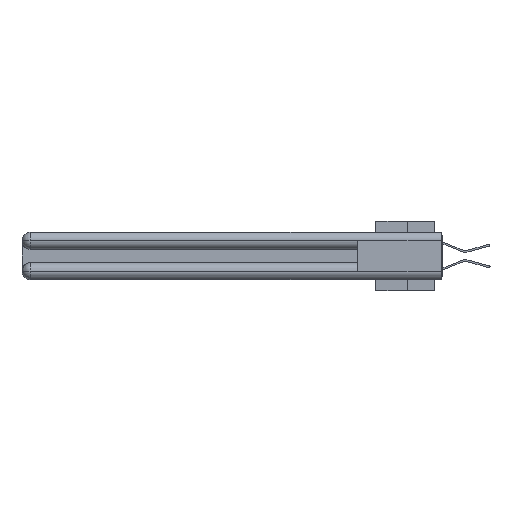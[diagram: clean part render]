
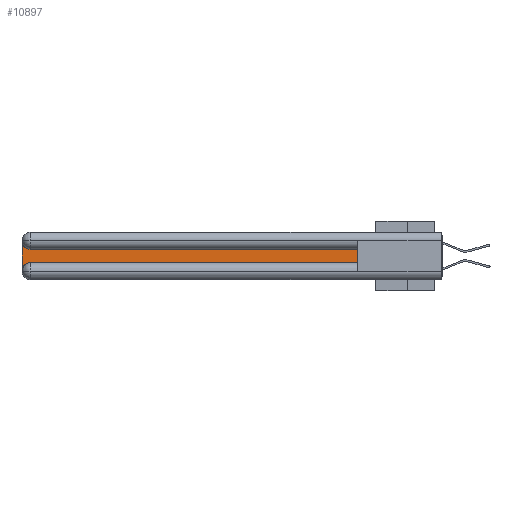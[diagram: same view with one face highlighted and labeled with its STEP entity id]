
A CAD part, left-side view. The second image highlights one B-rep face of the part: STEP entity #10897.
In plain terms, the highlighted planar face has unit normal (-1, 0, 0).
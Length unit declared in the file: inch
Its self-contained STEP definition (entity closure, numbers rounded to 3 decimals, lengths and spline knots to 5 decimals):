
#558 = PLANE ( 'NONE',  #18155 ) ;
#804 = DIRECTION ( 'NONE',  ( 1., 0., 0. ) ) ;
#1909 = VECTOR ( 'NONE', #27514, 39.37008 ) ;
#1958 = DIRECTION ( 'NONE',  ( 1., 0., 0. ) ) ;
#2050 = AXIS2_PLACEMENT_3D ( 'NONE', #28147, #11711, #31362 ) ;
#2185 = CARTESIAN_POINT ( 'NONE',  ( 0.075, 2.94, -0.0625 ) ) ;
#2773 = LINE ( 'NONE', #30263, #1909 ) ;
#3447 = DIRECTION ( 'NONE',  ( 0., 0., -1. ) ) ;
#4898 = CARTESIAN_POINT ( 'NONE',  ( 0.075, 2.94, -0.2175 ) ) ;
#7328 = DIRECTION ( 'NONE',  ( 0., -1., 0. ) ) ;
#7386 = CARTESIAN_POINT ( 'NONE',  ( 0.075, 0.6, -0.1225 ) ) ;
#7410 = CARTESIAN_POINT ( 'NONE',  ( 0.075, 2.94, -0.1225 ) ) ;
#7821 = CARTESIAN_POINT ( 'NONE',  ( 0.075, 0.6, -0.2175 ) ) ;
#8546 = EDGE_CURVE ( 'NONE', #30610, #24646, #12471, .T. ) ;
#9130 = VECTOR ( 'NONE', #7328, 39.37008 ) ;
#10398 = LINE ( 'NONE', #18314, #9130 ) ;
#10419 = ORIENTED_EDGE ( 'NONE', *, *, #33603, .T. ) ;
#10897 = ADVANCED_FACE ( 'NONE', ( #31747 ), #558, .F. ) ;
#11254 = EDGE_CURVE ( 'NONE', #23061, #30610, #17925, .T. ) ;
#11711 = DIRECTION ( 'NONE',  ( 1., 0., 0. ) ) ;
#12378 = ORIENTED_EDGE ( 'NONE', *, *, #11254, .T. ) ;
#12471 = CIRCLE ( 'NONE', #2050, 0.06 ) ;
#13074 = CARTESIAN_POINT ( 'NONE',  ( 0.075, 3., -0.2175 ) ) ;
#13587 = ORIENTED_EDGE ( 'NONE', *, *, #8546, .T. ) ;
#14089 = VECTOR ( 'NONE', #21341, 39.37008 ) ;
#15757 = AXIS2_PLACEMENT_3D ( 'NONE', #2185, #1958, #32156 ) ;
#16210 = DIRECTION ( 'NONE',  ( 0., 0., 1. ) ) ;
#16212 = VERTEX_POINT ( 'NONE', #7410 ) ;
#16827 = EDGE_CURVE ( 'NONE', #16212, #23061, #25061, .T. ) ;
#17368 = EDGE_CURVE ( 'NONE', #24646, #25975, #10398, .T. ) ;
#17925 = LINE ( 'NONE', #13074, #14089 ) ;
#18155 = AXIS2_PLACEMENT_3D ( 'NONE', #28028, #804, #3447 ) ;
#18314 = CARTESIAN_POINT ( 'NONE',  ( 0.075, 0.6, -0.2175 ) ) ;
#19332 = CARTESIAN_POINT ( 'NONE',  ( 0.075, 3., -0.2775 ) ) ;
#21341 = DIRECTION ( 'NONE',  ( 0., 0., -1. ) ) ;
#22394 = ORIENTED_EDGE ( 'NONE', *, *, #32527, .T. ) ;
#23061 = VERTEX_POINT ( 'NONE', #33480 ) ;
#23354 = VERTEX_POINT ( 'NONE', #7386 ) ;
#24646 = VERTEX_POINT ( 'NONE', #4898 ) ;
#25061 = CIRCLE ( 'NONE', #15757, 0.06 ) ;
#25975 = VERTEX_POINT ( 'NONE', #7821 ) ;
#26243 = ORIENTED_EDGE ( 'NONE', *, *, #17368, .T. ) ;
#26288 = LINE ( 'NONE', #27355, #31012 ) ;
#27355 = CARTESIAN_POINT ( 'NONE',  ( 0.075, 0.6, -0.2175 ) ) ;
#27514 = DIRECTION ( 'NONE',  ( 0., 1., 0. ) ) ;
#28028 = CARTESIAN_POINT ( 'NONE',  ( 0.075, 3., -0.1225 ) ) ;
#28147 = CARTESIAN_POINT ( 'NONE',  ( 0.075, 2.94, -0.2775 ) ) ;
#28623 = EDGE_LOOP ( 'NONE', ( #22394, #31004, #12378, #13587, #26243, #10419 ) ) ;
#30263 = CARTESIAN_POINT ( 'NONE',  ( 0.075, 0.6, -0.1225 ) ) ;
#30610 = VERTEX_POINT ( 'NONE', #19332 ) ;
#31004 = ORIENTED_EDGE ( 'NONE', *, *, #16827, .T. ) ;
#31012 = VECTOR ( 'NONE', #16210, 39.37008 ) ;
#31362 = DIRECTION ( 'NONE',  ( 0., 0., -1. ) ) ;
#31747 = FACE_OUTER_BOUND ( 'NONE', #28623, .T. ) ;
#32156 = DIRECTION ( 'NONE',  ( 0., 0., -1. ) ) ;
#32527 = EDGE_CURVE ( 'NONE', #23354, #16212, #2773, .T. ) ;
#33480 = CARTESIAN_POINT ( 'NONE',  ( 0.075, 3., -0.0625 ) ) ;
#33603 = EDGE_CURVE ( 'NONE', #25975, #23354, #26288, .T. ) ;
